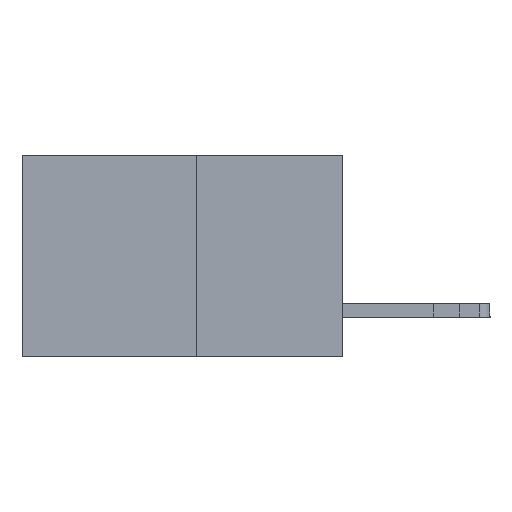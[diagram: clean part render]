
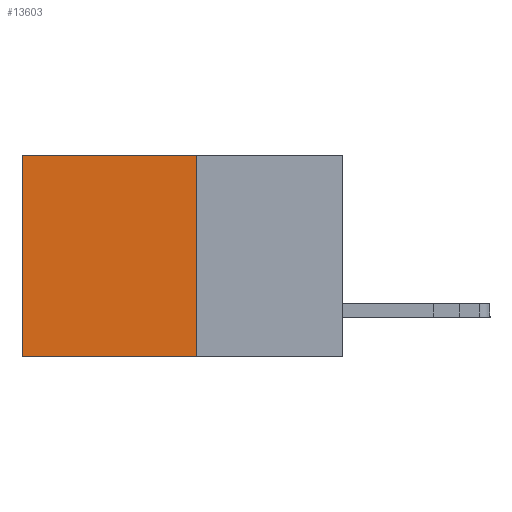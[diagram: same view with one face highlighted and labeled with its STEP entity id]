
A CAD part, left-side view. The second image highlights one B-rep face of the part: STEP entity #13603.
In plain terms, the highlighted planar face has unit normal (-1, 0, 0).
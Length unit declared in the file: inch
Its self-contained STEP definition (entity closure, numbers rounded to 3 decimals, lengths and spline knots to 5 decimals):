
#72 = EDGE_CURVE ( 'NONE', #18560, #8361, #2166, .T. ) ;
#676 = ORIENTED_EDGE ( 'NONE', *, *, #72, .F. ) ;
#2166 = LINE ( 'NONE', #6235, #10967 ) ;
#2542 = CARTESIAN_POINT ( 'NONE',  ( 0.277, 0.59, -0.37 ) ) ;
#2844 = CARTESIAN_POINT ( 'NONE',  ( 0.277, 0.27, -0.37 ) ) ;
#3485 = DIRECTION ( 'NONE',  ( 0., 0., -1. ) ) ;
#3869 = LINE ( 'NONE', #2542, #16082 ) ;
#4457 = DIRECTION ( 'NONE',  ( 0., 0., -1. ) ) ;
#6186 = EDGE_CURVE ( 'NONE', #17482, #18560, #16142, .T. ) ;
#6235 = CARTESIAN_POINT ( 'NONE',  ( 0.277, 0.27, -0.37 ) ) ;
#6256 = DIRECTION ( 'NONE',  ( 0., 1., 0. ) ) ;
#6378 = CARTESIAN_POINT ( 'NONE',  ( 0.277, 0.59, -0.37 ) ) ;
#6454 = VECTOR ( 'NONE', #19118, 39.37008 ) ;
#6619 = CARTESIAN_POINT ( 'NONE',  ( 0.277, 0.27, -0.37 ) ) ;
#7018 = CARTESIAN_POINT ( 'NONE',  ( 0.277, 0.27, 0. ) ) ;
#8361 = VERTEX_POINT ( 'NONE', #6378 ) ;
#8461 = ORIENTED_EDGE ( 'NONE', *, *, #8973, .T. ) ;
#8515 = ORIENTED_EDGE ( 'NONE', *, *, #18263, .T. ) ;
#8973 = EDGE_CURVE ( 'NONE', #10715, #8361, #3869, .T. ) ;
#9603 = EDGE_LOOP ( 'NONE', ( #8461, #676, #13850, #8515 ) ) ;
#10178 = CARTESIAN_POINT ( 'NONE',  ( 0.277, 0.27, 0. ) ) ;
#10715 = VERTEX_POINT ( 'NONE', #16809 ) ;
#10967 = VECTOR ( 'NONE', #6256, 39.37008 ) ;
#11585 = VECTOR ( 'NONE', #3485, 39.37008 ) ;
#13603 = ADVANCED_FACE ( 'NONE', ( #18323 ), #16483, .F. ) ;
#13850 = ORIENTED_EDGE ( 'NONE', *, *, #6186, .F. ) ;
#14784 = DIRECTION ( 'NONE',  ( 1., 0., 0. ) ) ;
#16082 = VECTOR ( 'NONE', #21682, 39.37008 ) ;
#16142 = LINE ( 'NONE', #6619, #11585 ) ;
#16483 = PLANE ( 'NONE',  #19313 ) ;
#16809 = CARTESIAN_POINT ( 'NONE',  ( 0.277, 0.59, 0. ) ) ;
#17482 = VERTEX_POINT ( 'NONE', #10178 ) ;
#18263 = EDGE_CURVE ( 'NONE', #17482, #10715, #18637, .T. ) ;
#18323 = FACE_OUTER_BOUND ( 'NONE', #9603, .T. ) ;
#18560 = VERTEX_POINT ( 'NONE', #2844 ) ;
#18637 = LINE ( 'NONE', #7018, #6454 ) ;
#19118 = DIRECTION ( 'NONE',  ( 0., 1., 0. ) ) ;
#19313 = AXIS2_PLACEMENT_3D ( 'NONE', #19986, #14784, #4457 ) ;
#19986 = CARTESIAN_POINT ( 'NONE',  ( 0.277, 0.27, -0.37 ) ) ;
#21682 = DIRECTION ( 'NONE',  ( 0., 0., -1. ) ) ;
